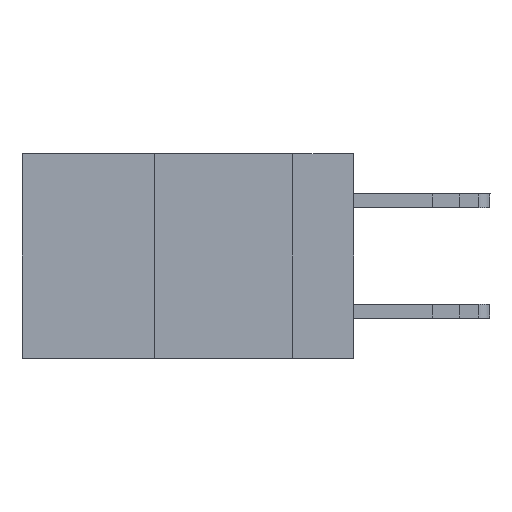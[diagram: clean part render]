
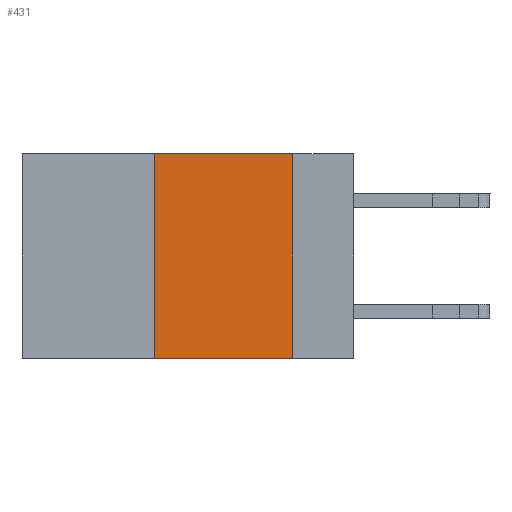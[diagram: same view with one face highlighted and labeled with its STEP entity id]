
A CAD part, left-side view. The second image highlights one B-rep face of the part: STEP entity #431.
In plain terms, the highlighted planar face has unit normal (-1, 0, 0).
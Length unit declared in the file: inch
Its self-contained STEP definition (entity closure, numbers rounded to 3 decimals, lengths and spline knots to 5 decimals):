
#431 = ADVANCED_FACE ( 'NONE', ( #2694 ), #6361, .F. ) ;
#641 = DIRECTION ( 'NONE',  ( 0., -1., 0. ) ) ;
#813 = LINE ( 'NONE', #3664, #8493 ) ;
#925 = EDGE_CURVE ( 'NONE', #11184, #14609, #5588, .T. ) ;
#1649 = LINE ( 'NONE', #15119, #7940 ) ;
#2220 = VECTOR ( 'NONE', #13545, 39.37008 ) ;
#2694 = FACE_OUTER_BOUND ( 'NONE', #5964, .T. ) ;
#3519 = VERTEX_POINT ( 'NONE', #13670 ) ;
#3664 = CARTESIAN_POINT ( 'NONE',  ( 0., 0.6, -0.37 ) ) ;
#3665 = EDGE_CURVE ( 'NONE', #14609, #16696, #1649, .T. ) ;
#4820 = LINE ( 'NONE', #8550, #12008 ) ;
#5050 = ORIENTED_EDGE ( 'NONE', *, *, #925, .F. ) ;
#5252 = ORIENTED_EDGE ( 'NONE', *, *, #17235, .T. ) ;
#5292 = DIRECTION ( 'NONE',  ( 1., 0., 0. ) ) ;
#5588 = LINE ( 'NONE', #11917, #2220 ) ;
#5964 = EDGE_LOOP ( 'NONE', ( #6076, #5050, #17695, #5252 ) ) ;
#6076 = ORIENTED_EDGE ( 'NONE', *, *, #3665, .F. ) ;
#6361 = PLANE ( 'NONE',  #17551 ) ;
#7940 = VECTOR ( 'NONE', #7968, 39.37008 ) ;
#7968 = DIRECTION ( 'NONE',  ( 0., 0., -1. ) ) ;
#8291 = DIRECTION ( 'NONE',  ( 0., 0., 1. ) ) ;
#8493 = VECTOR ( 'NONE', #641, 39.37008 ) ;
#8550 = CARTESIAN_POINT ( 'NONE',  ( 0., 0.36, 0. ) ) ;
#9331 = CARTESIAN_POINT ( 'NONE',  ( 0., 0.11, 0. ) ) ;
#11184 = VERTEX_POINT ( 'NONE', #12067 ) ;
#11917 = CARTESIAN_POINT ( 'NONE',  ( 0., 0.6, 0. ) ) ;
#12008 = VECTOR ( 'NONE', #8291, 39.37008 ) ;
#12067 = CARTESIAN_POINT ( 'NONE',  ( 0., 0.36, 0. ) ) ;
#12413 = CARTESIAN_POINT ( 'NONE',  ( 0., 0.11, -0.37 ) ) ;
#13545 = DIRECTION ( 'NONE',  ( 0., -1., 0. ) ) ;
#13670 = CARTESIAN_POINT ( 'NONE',  ( 0., 0.36, -0.37 ) ) ;
#14078 = EDGE_CURVE ( 'NONE', #3519, #11184, #4820, .T. ) ;
#14609 = VERTEX_POINT ( 'NONE', #9331 ) ;
#15119 = CARTESIAN_POINT ( 'NONE',  ( 0., 0.11, 0. ) ) ;
#15329 = DIRECTION ( 'NONE',  ( 0., 0., -1. ) ) ;
#16415 = CARTESIAN_POINT ( 'NONE',  ( 0., 0.6, 0. ) ) ;
#16696 = VERTEX_POINT ( 'NONE', #12413 ) ;
#17235 = EDGE_CURVE ( 'NONE', #3519, #16696, #813, .T. ) ;
#17551 = AXIS2_PLACEMENT_3D ( 'NONE', #16415, #5292, #15329 ) ;
#17695 = ORIENTED_EDGE ( 'NONE', *, *, #14078, .F. ) ;
